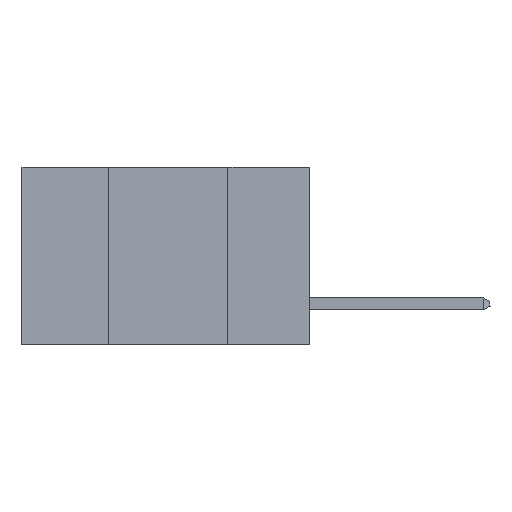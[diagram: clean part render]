
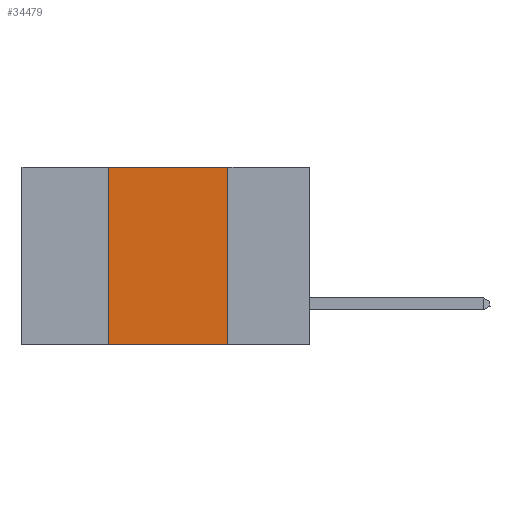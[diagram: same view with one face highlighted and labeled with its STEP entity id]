
A CAD part, left-side view. The second image highlights one B-rep face of the part: STEP entity #34479.
In plain terms, the highlighted planar face has unit normal (-1, 0, 0).
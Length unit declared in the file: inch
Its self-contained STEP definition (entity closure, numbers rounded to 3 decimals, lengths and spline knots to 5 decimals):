
#4154 = CARTESIAN_POINT ( 'NONE',  ( 0., 0.17, 0. ) ) ;
#4376 = CARTESIAN_POINT ( 'NONE',  ( 0., 0.42, -0.37 ) ) ;
#4959 = CARTESIAN_POINT ( 'NONE',  ( 0., 0.6, 0. ) ) ;
#6125 = LINE ( 'NONE', #4154, #15579 ) ;
#7280 = CARTESIAN_POINT ( 'NONE',  ( 0., 0.6, 0. ) ) ;
#10097 = LINE ( 'NONE', #21783, #24085 ) ;
#10304 = VECTOR ( 'NONE', #34393, 39.37008 ) ;
#10417 = FACE_OUTER_BOUND ( 'NONE', #19438, .T. ) ;
#11618 = VERTEX_POINT ( 'NONE', #28238 ) ;
#11824 = EDGE_CURVE ( 'NONE', #23437, #11618, #6125, .T. ) ;
#13161 = DIRECTION ( 'NONE',  ( 0., 0., -1. ) ) ;
#13425 = LINE ( 'NONE', #7280, #34359 ) ;
#13633 = PLANE ( 'NONE',  #24968 ) ;
#14513 = EDGE_CURVE ( 'NONE', #32016, #31447, #10097, .T. ) ;
#15579 = VECTOR ( 'NONE', #32246, 39.37008 ) ;
#15962 = DIRECTION ( 'NONE',  ( 0., -1., 0. ) ) ;
#19093 = CARTESIAN_POINT ( 'NONE',  ( 0., 0.42, 0. ) ) ;
#19438 = EDGE_LOOP ( 'NONE', ( #20301, #26206, #23156, #27669 ) ) ;
#20102 = CARTESIAN_POINT ( 'NONE',  ( 0., 0.17, 0. ) ) ;
#20301 = ORIENTED_EDGE ( 'NONE', *, *, #11824, .F. ) ;
#21783 = CARTESIAN_POINT ( 'NONE',  ( 0., 0.42, 0. ) ) ;
#22941 = EDGE_CURVE ( 'NONE', #32016, #11618, #27785, .T. ) ;
#23156 = ORIENTED_EDGE ( 'NONE', *, *, #14513, .F. ) ;
#23437 = VERTEX_POINT ( 'NONE', #20102 ) ;
#24085 = VECTOR ( 'NONE', #28076, 39.37008 ) ;
#24968 = AXIS2_PLACEMENT_3D ( 'NONE', #4959, #32921, #13161 ) ;
#25978 = CARTESIAN_POINT ( 'NONE',  ( 0., 0.6, -0.37 ) ) ;
#26206 = ORIENTED_EDGE ( 'NONE', *, *, #27305, .F. ) ;
#27305 = EDGE_CURVE ( 'NONE', #31447, #23437, #13425, .T. ) ;
#27669 = ORIENTED_EDGE ( 'NONE', *, *, #22941, .T. ) ;
#27785 = LINE ( 'NONE', #25978, #10304 ) ;
#28076 = DIRECTION ( 'NONE',  ( 0., 0., 1. ) ) ;
#28238 = CARTESIAN_POINT ( 'NONE',  ( 0., 0.17, -0.37 ) ) ;
#31447 = VERTEX_POINT ( 'NONE', #19093 ) ;
#32016 = VERTEX_POINT ( 'NONE', #4376 ) ;
#32246 = DIRECTION ( 'NONE',  ( 0., 0., -1. ) ) ;
#32921 = DIRECTION ( 'NONE',  ( 1., 0., 0. ) ) ;
#34359 = VECTOR ( 'NONE', #15962, 39.37008 ) ;
#34393 = DIRECTION ( 'NONE',  ( 0., -1., 0. ) ) ;
#34479 = ADVANCED_FACE ( 'NONE', ( #10417 ), #13633, .F. ) ;
